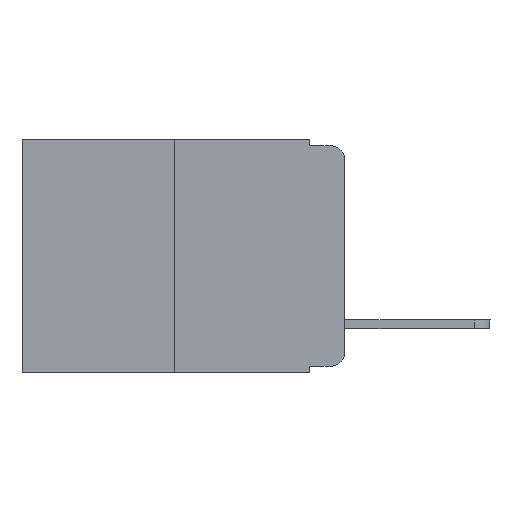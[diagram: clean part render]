
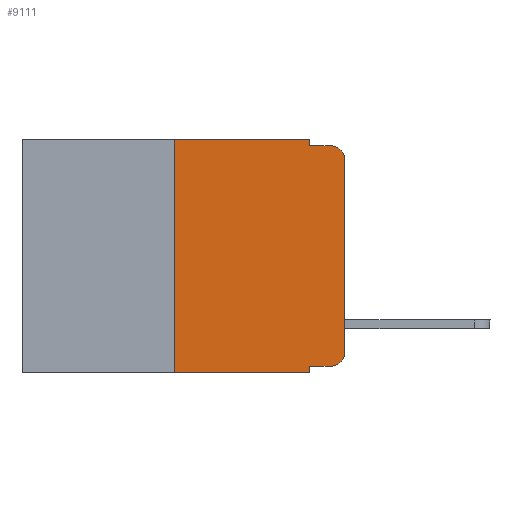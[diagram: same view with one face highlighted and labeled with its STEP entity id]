
A CAD part, left-side view. The second image highlights one B-rep face of the part: STEP entity #9111.
In plain terms, the highlighted planar face has unit normal (-1, 0, 0).
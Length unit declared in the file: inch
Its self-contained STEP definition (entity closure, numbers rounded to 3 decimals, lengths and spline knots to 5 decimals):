
#150 = VECTOR ( 'NONE', #3105, 39.37008 ) ;
#187 = CARTESIAN_POINT ( 'NONE',  ( 0., 0., 0. ) ) ;
#240 = CARTESIAN_POINT ( 'NONE',  ( 0., 0.473, 0. ) ) ;
#462 = VERTEX_POINT ( 'NONE', #695 ) ;
#547 = DIRECTION ( 'NONE',  ( -1., 0., 0. ) ) ;
#695 = CARTESIAN_POINT ( 'NONE',  ( 0., 0., -0.313 ) ) ;
#812 = EDGE_CURVE ( 'NONE', #13594, #17435, #17642, .T. ) ;
#1174 = CARTESIAN_POINT ( 'NONE',  ( 0., 0.473, 0. ) ) ;
#1517 = AXIS2_PLACEMENT_3D ( 'NONE', #7903, #15366, #1839 ) ;
#1641 = CARTESIAN_POINT ( 'NONE',  ( 0., 0.25, -0.343 ) ) ;
#1822 = EDGE_CURVE ( 'NONE', #10166, #13594, #2486, .T. ) ;
#1839 = DIRECTION ( 'NONE',  ( 0., 0., -1. ) ) ;
#2040 = AXIS2_PLACEMENT_3D ( 'NONE', #240, #7815, #13602 ) ;
#2486 = LINE ( 'NONE', #1174, #8823 ) ;
#2639 = DIRECTION ( 'NONE',  ( 0., -1., 0. ) ) ;
#2655 = EDGE_CURVE ( 'NONE', #462, #6462, #5007, .T. ) ;
#3105 = DIRECTION ( 'NONE',  ( 0., -1., 0. ) ) ;
#3227 = ORIENTED_EDGE ( 'NONE', *, *, #19357, .T. ) ;
#3248 = DIRECTION ( 'NONE',  ( 0., 0., -1. ) ) ;
#3399 = VECTOR ( 'NONE', #14563, 39.37008 ) ;
#3890 = ORIENTED_EDGE ( 'NONE', *, *, #11026, .T. ) ;
#3970 = EDGE_LOOP ( 'NONE', ( #9961, #12066, #11261, #5551, #7321, #10363, #3227, #14458, #6408, #3890 ) ) ;
#4203 = CARTESIAN_POINT ( 'NONE',  ( 0., 0.02, -0.333 ) ) ;
#4596 = LINE ( 'NONE', #10479, #14032 ) ;
#4909 = CARTESIAN_POINT ( 'NONE',  ( 0., 0.02, -0.03 ) ) ;
#5007 = LINE ( 'NONE', #187, #18945 ) ;
#5044 = LINE ( 'NONE', #12754, #3399 ) ;
#5121 = VECTOR ( 'NONE', #11788, 39.37008 ) ;
#5299 = VECTOR ( 'NONE', #12462, 39.37008 ) ;
#5551 = ORIENTED_EDGE ( 'NONE', *, *, #812, .F. ) ;
#5903 = AXIS2_PLACEMENT_3D ( 'NONE', #4909, #547, #17177 ) ;
#6100 = CARTESIAN_POINT ( 'NONE',  ( 0., 0.051, -0.333 ) ) ;
#6192 = CIRCLE ( 'NONE', #5903, 0.02 ) ;
#6250 = EDGE_CURVE ( 'NONE', #6462, #14806, #6192, .T. ) ;
#6408 = ORIENTED_EDGE ( 'NONE', *, *, #19133, .T. ) ;
#6462 = VERTEX_POINT ( 'NONE', #17307 ) ;
#6555 = CARTESIAN_POINT ( 'NONE',  ( 0., 0.473, -0.343 ) ) ;
#6764 = CIRCLE ( 'NONE', #1517, 0.02 ) ;
#7075 = FACE_OUTER_BOUND ( 'NONE', #3970, .T. ) ;
#7321 = ORIENTED_EDGE ( 'NONE', *, *, #1822, .F. ) ;
#7535 = DIRECTION ( 'NONE',  ( 0., -1., 0. ) ) ;
#7815 = DIRECTION ( 'NONE',  ( 1., 0., 0. ) ) ;
#7903 = CARTESIAN_POINT ( 'NONE',  ( 0., 0.02, -0.313 ) ) ;
#8823 = VECTOR ( 'NONE', #2639, 39.37008 ) ;
#9111 = ADVANCED_FACE ( 'NONE', ( #7075 ), #13668, .F. ) ;
#9484 = CARTESIAN_POINT ( 'NONE',  ( 0., 0.051, 0. ) ) ;
#9779 = LINE ( 'NONE', #6555, #5299 ) ;
#9961 = ORIENTED_EDGE ( 'NONE', *, *, #2655, .T. ) ;
#10139 = LINE ( 'NONE', #9484, #17724 ) ;
#10166 = VERTEX_POINT ( 'NONE', #10629 ) ;
#10328 = EDGE_CURVE ( 'NONE', #17435, #14806, #14085, .T. ) ;
#10363 = ORIENTED_EDGE ( 'NONE', *, *, #14561, .F. ) ;
#10479 = CARTESIAN_POINT ( 'NONE',  ( 0., 0.051, -0.333 ) ) ;
#10629 = CARTESIAN_POINT ( 'NONE',  ( 0., 0.25, 0. ) ) ;
#11026 = EDGE_CURVE ( 'NONE', #14566, #462, #6764, .T. ) ;
#11261 = ORIENTED_EDGE ( 'NONE', *, *, #10328, .F. ) ;
#11788 = DIRECTION ( 'NONE',  ( 0., 0., -1. ) ) ;
#11998 = CARTESIAN_POINT ( 'NONE',  ( 0., 0.051, 0. ) ) ;
#12066 = ORIENTED_EDGE ( 'NONE', *, *, #6250, .T. ) ;
#12462 = DIRECTION ( 'NONE',  ( 0., -1., 0. ) ) ;
#12754 = CARTESIAN_POINT ( 'NONE',  ( 0., 0.25, 0. ) ) ;
#13594 = VERTEX_POINT ( 'NONE', #11998 ) ;
#13602 = DIRECTION ( 'NONE',  ( 0., 0., -1. ) ) ;
#13668 = PLANE ( 'NONE',  #2040 ) ;
#13801 = CARTESIAN_POINT ( 'NONE',  ( 0., 0.02, -0.01 ) ) ;
#14032 = VECTOR ( 'NONE', #7535, 39.37008 ) ;
#14085 = LINE ( 'NONE', #15303, #150 ) ;
#14263 = VERTEX_POINT ( 'NONE', #6100 ) ;
#14458 = ORIENTED_EDGE ( 'NONE', *, *, #17178, .F. ) ;
#14561 = EDGE_CURVE ( 'NONE', #18054, #10166, #5044, .T. ) ;
#14563 = DIRECTION ( 'NONE',  ( 0., 0., 1. ) ) ;
#14566 = VERTEX_POINT ( 'NONE', #4203 ) ;
#14769 = CARTESIAN_POINT ( 'NONE',  ( 0., 0.051, 0. ) ) ;
#14806 = VERTEX_POINT ( 'NONE', #13801 ) ;
#15303 = CARTESIAN_POINT ( 'NONE',  ( 0., 0.051, -0.01 ) ) ;
#15366 = DIRECTION ( 'NONE',  ( -1., 0., 0. ) ) ;
#16805 = DIRECTION ( 'NONE',  ( 0., 0., 1. ) ) ;
#17177 = DIRECTION ( 'NONE',  ( 0., 0., -1. ) ) ;
#17178 = EDGE_CURVE ( 'NONE', #14263, #17725, #10139, .T. ) ;
#17307 = CARTESIAN_POINT ( 'NONE',  ( 0., 0., -0.03 ) ) ;
#17435 = VERTEX_POINT ( 'NONE', #17494 ) ;
#17494 = CARTESIAN_POINT ( 'NONE',  ( 0., 0.051, -0.01 ) ) ;
#17642 = LINE ( 'NONE', #14769, #5121 ) ;
#17649 = CARTESIAN_POINT ( 'NONE',  ( 0., 0.051, -0.343 ) ) ;
#17724 = VECTOR ( 'NONE', #3248, 39.37008 ) ;
#17725 = VERTEX_POINT ( 'NONE', #17649 ) ;
#18054 = VERTEX_POINT ( 'NONE', #1641 ) ;
#18945 = VECTOR ( 'NONE', #16805, 39.37008 ) ;
#19133 = EDGE_CURVE ( 'NONE', #14263, #14566, #4596, .T. ) ;
#19357 = EDGE_CURVE ( 'NONE', #18054, #17725, #9779, .T. ) ;
